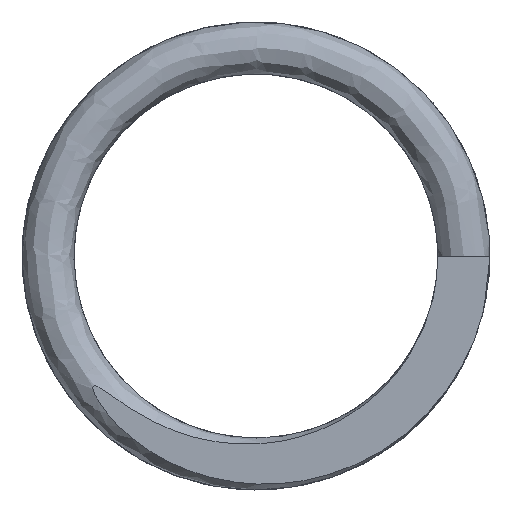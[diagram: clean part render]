
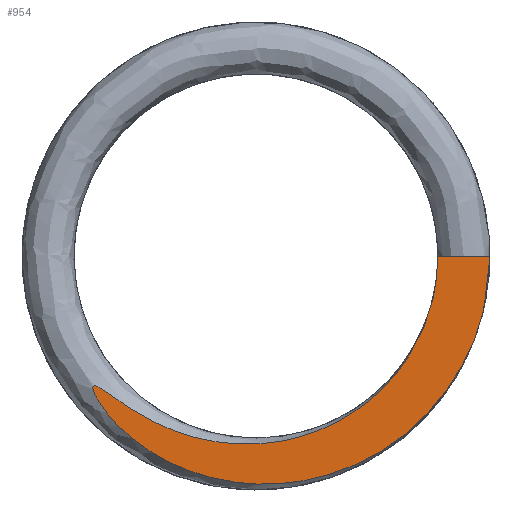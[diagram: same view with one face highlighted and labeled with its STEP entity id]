
A CAD part, front view. The second image highlights one B-rep face of the part: STEP entity #954.
In plain terms, the highlighted planar face has unit normal (0, -1, 0).
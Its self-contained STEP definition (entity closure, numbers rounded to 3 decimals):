
#4 = CARTESIAN_POINT ( 'NONE',  ( -1.546, 0., -1.347 ) ) ;
#63 = CARTESIAN_POINT ( 'NONE',  ( -1.119, 0., -1.523 ) ) ;
#144 = AXIS2_PLACEMENT_3D ( 'NONE', #1565, #317, #1772 ) ;
#149 = CARTESIAN_POINT ( 'NONE',  ( 1.738, 0., -0.208 ) ) ;
#195 = CARTESIAN_POINT ( 'NONE',  ( 0.826, 0., -2.069 ) ) ;
#203 = CARTESIAN_POINT ( 'NONE',  ( -1.57, 0., -1.271 ) ) ;
#317 = DIRECTION ( 'NONE',  ( 0., -1., 0. ) ) ;
#331 = CARTESIAN_POINT ( 'NONE',  ( -1.295, 0., -1.411 ) ) ;
#356 = CARTESIAN_POINT ( 'NONE',  ( -0.134, 0., -1.82 ) ) ;
#395 = CARTESIAN_POINT ( 'NONE',  ( 2.25, 0., 0. ) ) ;
#404 = CARTESIAN_POINT ( 'NONE',  ( 0.225, 0., -2.199 ) ) ;
#413 = CARTESIAN_POINT ( 'NONE',  ( -1.558, 0., -1.247 ) ) ;
#597 = CARTESIAN_POINT ( 'NONE',  ( 2.238, 0., -0.206 ) ) ;
#605 = CARTESIAN_POINT ( 'NONE',  ( -0.39, 0., -2.151 ) ) ;
#615 = CARTESIAN_POINT ( 'NONE',  ( -1.539, 0., -1.248 ) ) ;
#713 = CARTESIAN_POINT ( 'NONE',  ( 1.75, 0., 0. ) ) ;
#811 = CARTESIAN_POINT ( 'NONE',  ( 2.193, 0., -0.513 ) ) ;
#820 = EDGE_CURVE ( 'NONE', #1233, #1689, #1257, .T. ) ;
#821 = CARTESIAN_POINT ( 'NONE',  ( -0.964, 0., -1.924 ) ) ;
#831 = CARTESIAN_POINT ( 'NONE',  ( -1.486, 0., -1.275 ) ) ;
#849 = CARTESIAN_POINT ( 'NONE',  ( 2., 0., 0. ) ) ;
#869 = LINE ( 'NONE', #849, #944 ) ;
#929 = CARTESIAN_POINT ( 'NONE',  ( 1.57, 0., -0.808 ) ) ;
#944 = VECTOR ( 'NONE', #2287, 1000. ) ;
#954 = ADVANCED_FACE ( 'NONE', ( #968 ), #1355, .T. ) ;
#968 = FACE_OUTER_BOUND ( 'NONE', #1341, .T. ) ;
#1008 = CARTESIAN_POINT ( 'NONE',  ( -0.544, 0., -1.766 ) ) ;
#1026 = CARTESIAN_POINT ( 'NONE',  ( 2.023, 0., -0.996 ) ) ;
#1036 = CARTESIAN_POINT ( 'NONE',  ( -1.362, 0., -1.597 ) ) ;
#1071 = EDGE_CURVE ( 'NONE', #1233, #1689, #869, .T. ) ;
#1077 = CARTESIAN_POINT ( 'NONE',  ( 1.038, 0., -1.447 ) ) ;
#1098 = CARTESIAN_POINT ( 'NONE',  ( 0.078, 0., -1.813 ) ) ;
#1150 = CARTESIAN_POINT ( 'NONE',  ( -0.747, 0., -1.705 ) ) ;
#1231 = CARTESIAN_POINT ( 'NONE',  ( 1.673, 0., -1.502 ) ) ;
#1233 = VERTEX_POINT ( 'NONE', #2540 ) ;
#1241 = CARTESIAN_POINT ( 'NONE',  ( -1.518, 0., -1.391 ) ) ;
#1257 = B_SPLINE_CURVE_WITH_KNOTS ( 'NONE', 3,
 ( #713, #1766, #149, #2584, #2208, #929, #2625, #2543, #1077, #1588, #1601, #1098, #356, #1008, #1150, #1594, #63, #331, #2060, #831, #2269, #615, #1862, #413, #1663, #203, #1449, #4, #1241, #2462, #1036, #2260, #821, #2049, #605, #1852, #404, #1654, #195, #1441, #2651, #1231, #2454, #1026, #2250, #811, #2041, #597, #1843, #395 ),
 .UNSPECIFIED., .F., .F.,
 ( 4, 2, 2, 2, 2, 2, 2, 2, 2, 2, 2, 2, 2, 2, 2, 2, 2, 2, 2, 2, 2, 2, 2, 2, 4 ),
 ( 0., 0., 0.001, 0.001, 0.002, 0.002, 0.003, 0.004, 0.004, 0.004, 0.004, 0.004, 0.004, 0.005, 0.005, 0.005, 0.006, 0.006, 0.007, 0.007, 0.008, 0.009, 0.009, 0.01, 0.01 ),
 .UNSPECIFIED. ) ;
#1341 = EDGE_LOOP ( 'NONE', ( #1571, #1572 ) ) ;
#1355 = PLANE ( 'NONE',  #144 ) ;
#1441 = CARTESIAN_POINT ( 'NONE',  ( 1.195, 0., -1.892 ) ) ;
#1449 = CARTESIAN_POINT ( 'NONE',  ( -1.566, 0., -1.284 ) ) ;
#1565 = CARTESIAN_POINT ( 'NONE',  ( 0., 0., -2.25 ) ) ;
#1571 = ORIENTED_EDGE ( 'NONE', *, *, #820, .T. ) ;
#1572 = ORIENTED_EDGE ( 'NONE', *, *, #1071, .F. ) ;
#1588 = CARTESIAN_POINT ( 'NONE',  ( 0.682, 0., -1.657 ) ) ;
#1594 = CARTESIAN_POINT ( 'NONE',  ( -1.029, 0., -1.573 ) ) ;
#1601 = CARTESIAN_POINT ( 'NONE',  ( 0.483, 0., -1.733 ) ) ;
#1654 = CARTESIAN_POINT ( 'NONE',  ( 0.628, 0., -2.133 ) ) ;
#1663 = CARTESIAN_POINT ( 'NONE',  ( -1.564, 0., -1.252 ) ) ;
#1689 = VERTEX_POINT ( 'NONE', #1740 ) ;
#1740 = CARTESIAN_POINT ( 'NONE',  ( 2.25, 0., 0. ) ) ;
#1766 = CARTESIAN_POINT ( 'NONE',  ( 1.744, 0., -0.104 ) ) ;
#1772 = DIRECTION ( 'NONE',  ( 0., 0., -1. ) ) ;
#1843 = CARTESIAN_POINT ( 'NONE',  ( 2.244, 0., -0.103 ) ) ;
#1852 = CARTESIAN_POINT ( 'NONE',  ( 0.015, 0., -2.203 ) ) ;
#1862 = CARTESIAN_POINT ( 'NONE',  ( -1.545, 0., -1.247 ) ) ;
#2041 = CARTESIAN_POINT ( 'NONE',  ( 2.213, 0., -0.411 ) ) ;
#2049 = CARTESIAN_POINT ( 'NONE',  ( -0.591, 0., -2.094 ) ) ;
#2060 = CARTESIAN_POINT ( 'NONE',  ( -1.378, 0., -1.348 ) ) ;
#2208 = CARTESIAN_POINT ( 'NONE',  ( 1.678, 0., -0.515 ) ) ;
#2250 = CARTESIAN_POINT ( 'NONE',  ( 2.108, 0., -0.809 ) ) ;
#2260 = CARTESIAN_POINT ( 'NONE',  ( -1.139, 0., -1.808 ) ) ;
#2269 = CARTESIAN_POINT ( 'NONE',  ( -1.508, 0., -1.26 ) ) ;
#2287 = DIRECTION ( 'NONE',  ( 1., 0., 0. ) ) ;
#2454 = CARTESIAN_POINT ( 'NONE',  ( 1.804, 0., -1.346 ) ) ;
#2462 = CARTESIAN_POINT ( 'NONE',  ( -1.431, 0., -1.52 ) ) ;
#2540 = CARTESIAN_POINT ( 'NONE',  ( 1.75, 0., 0. ) ) ;
#2543 = CARTESIAN_POINT ( 'NONE',  ( 1.2, 0., -1.31 ) ) ;
#2584 = CARTESIAN_POINT ( 'NONE',  ( 1.706, 0., -0.413 ) ) ;
#2625 = CARTESIAN_POINT ( 'NONE',  ( 1.465, 0., -0.992 ) ) ;
#2651 = CARTESIAN_POINT ( 'NONE',  ( 1.367, 0., -1.777 ) ) ;
